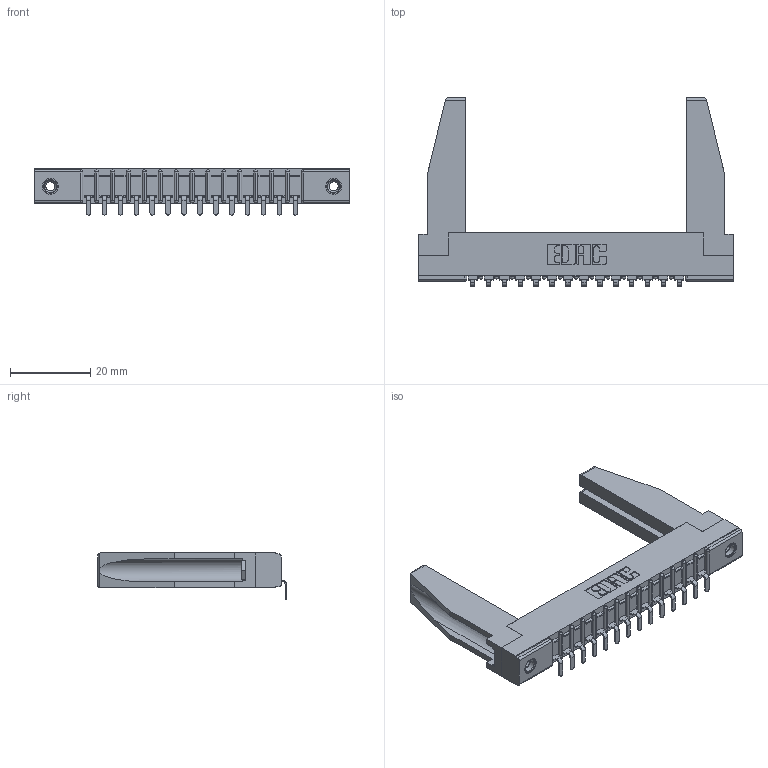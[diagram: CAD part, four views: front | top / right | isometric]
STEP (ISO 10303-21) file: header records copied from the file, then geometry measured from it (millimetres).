
FILE_DESCRIPTION (( 'STEP AP203' ), '1' );
FILE_NAME ('307-014-453-178.STEP', '2020-09-25T16:02:24', ( '' ), ( '' ), 'SwSTEP 2.0', 'SolidWorks 2020', '' );
FILE_SCHEMA (( 'CONFIG_CONTROL_DESIGN' ));
Length unit declared in the file: inch
Products named in the file (5): 307-220-078; 307 Part_.156 Dia Mounting Holes; 307-014-453-178; 307-290-002_553; 345-250-001_345-250-001-102
Assembly tree (19 placements, depth 2):
  307-014-453-178
    307 Part_.156 Dia Mounting Holes
    307-290-002_553  x14
    307-220-078  x2
    345-250-001_345-250-001-102  x2
Bounding box: 78.49 x 47.03 x 11.51 mm (x, y, z)
Volume: 9170.6 mm3; surface area: 12796.7 mm2
Topology: 19 solids, 19 shells, 1355 faces, 4069 edges, 2662 vertices
Faces by surface type: plane 812, cylinder 497, sphere 30, cone 12, torus 4
Entity records: 18747 total; most frequent: CARTESIAN_POINT 3158, ORIENTED_EDGE 3104, DIRECTION 3038, EDGE_CURVE 1552, LINE 1178, VECTOR 1178, VERTEX_POINT 1008, AXIS2_PLACEMENT_3D 930
